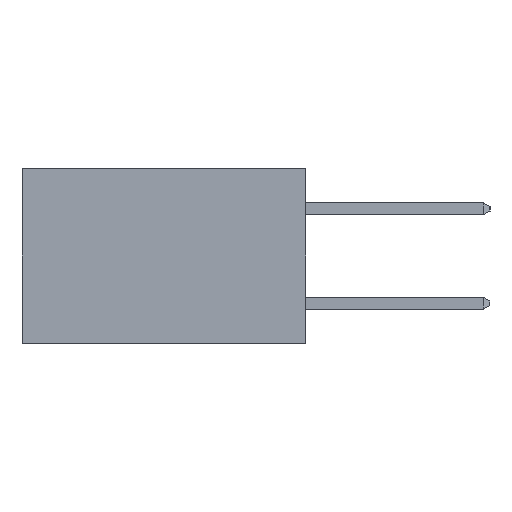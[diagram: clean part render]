
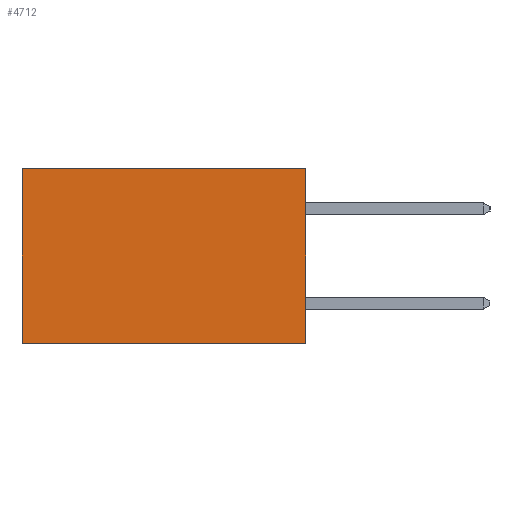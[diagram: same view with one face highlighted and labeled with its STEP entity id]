
A CAD part, left-side view. The second image highlights one B-rep face of the part: STEP entity #4712.
In plain terms, the highlighted planar face has unit normal (-1, 0, 0).
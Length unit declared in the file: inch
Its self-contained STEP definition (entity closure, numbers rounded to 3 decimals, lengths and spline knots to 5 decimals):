
#174 = ORIENTED_EDGE ( 'NONE', *, *, #6789, .T. ) ;
#271 = CARTESIAN_POINT ( 'NONE',  ( 0.298, 0., 0. ) ) ;
#797 = CARTESIAN_POINT ( 'NONE',  ( 0.298, 0., -0.37 ) ) ;
#1233 = VERTEX_POINT ( 'NONE', #4661 ) ;
#1260 = AXIS2_PLACEMENT_3D ( 'NONE', #9056, #6961, #7728 ) ;
#1602 = CARTESIAN_POINT ( 'NONE',  ( 0.298, 0., -0.37 ) ) ;
#1810 = VECTOR ( 'NONE', #10606, 39.37008 ) ;
#1993 = CARTESIAN_POINT ( 'NONE',  ( 0.298, 0.6, -0.37 ) ) ;
#2369 = EDGE_CURVE ( 'NONE', #3923, #1233, #4551, .T. ) ;
#3923 = VERTEX_POINT ( 'NONE', #13466 ) ;
#4372 = EDGE_CURVE ( 'NONE', #3923, #7549, #11838, .T. ) ;
#4551 = LINE ( 'NONE', #271, #7221 ) ;
#4661 = CARTESIAN_POINT ( 'NONE',  ( 0.298, 0.6, 0. ) ) ;
#4712 = ADVANCED_FACE ( 'NONE', ( #10376 ), #8834, .F. ) ;
#5676 = CARTESIAN_POINT ( 'NONE',  ( 0.298, 0., 0. ) ) ;
#6756 = LINE ( 'NONE', #7764, #8972 ) ;
#6789 = EDGE_CURVE ( 'NONE', #1233, #12496, #6756, .T. ) ;
#6961 = DIRECTION ( 'NONE',  ( 1., 0., 0. ) ) ;
#7156 = ORIENTED_EDGE ( 'NONE', *, *, #2369, .T. ) ;
#7221 = VECTOR ( 'NONE', #9357, 39.37008 ) ;
#7549 = VERTEX_POINT ( 'NONE', #797 ) ;
#7666 = DIRECTION ( 'NONE',  ( 0., 0., -1. ) ) ;
#7728 = DIRECTION ( 'NONE',  ( 0., 0., -1. ) ) ;
#7764 = CARTESIAN_POINT ( 'NONE',  ( 0.298, 0.6, 0. ) ) ;
#8303 = EDGE_LOOP ( 'NONE', ( #174, #8836, #9681, #7156 ) ) ;
#8834 = PLANE ( 'NONE',  #1260 ) ;
#8836 = ORIENTED_EDGE ( 'NONE', *, *, #13795, .F. ) ;
#8972 = VECTOR ( 'NONE', #7666, 39.37008 ) ;
#9045 = VECTOR ( 'NONE', #9897, 39.37008 ) ;
#9056 = CARTESIAN_POINT ( 'NONE',  ( 0.298, 0., 0. ) ) ;
#9357 = DIRECTION ( 'NONE',  ( 0., 1., 0. ) ) ;
#9681 = ORIENTED_EDGE ( 'NONE', *, *, #4372, .F. ) ;
#9897 = DIRECTION ( 'NONE',  ( 0., 0., -1. ) ) ;
#10376 = FACE_OUTER_BOUND ( 'NONE', #8303, .T. ) ;
#10606 = DIRECTION ( 'NONE',  ( 0., 1., 0. ) ) ;
#10781 = LINE ( 'NONE', #1602, #1810 ) ;
#11838 = LINE ( 'NONE', #5676, #9045 ) ;
#12496 = VERTEX_POINT ( 'NONE', #1993 ) ;
#13466 = CARTESIAN_POINT ( 'NONE',  ( 0.298, 0., 0. ) ) ;
#13795 = EDGE_CURVE ( 'NONE', #7549, #12496, #10781, .T. ) ;
